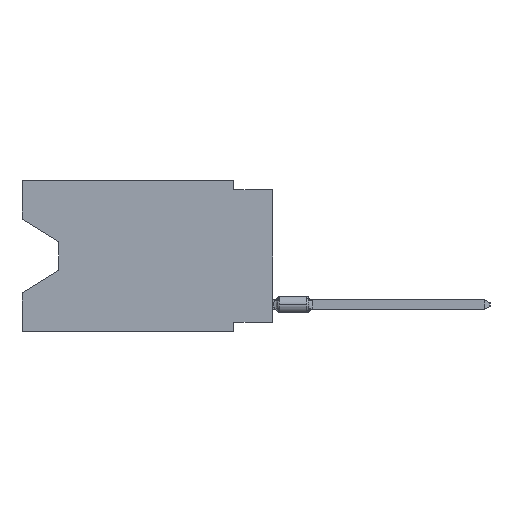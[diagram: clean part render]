
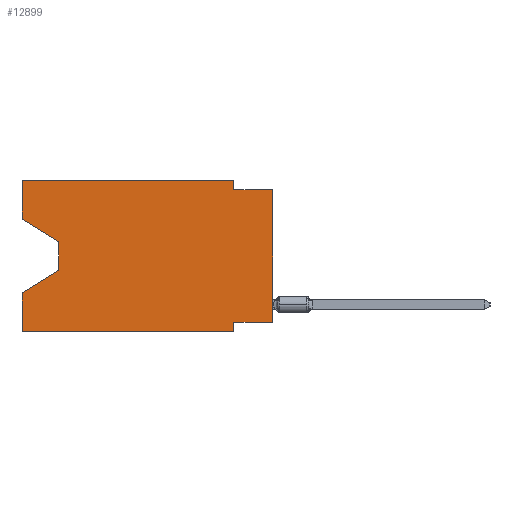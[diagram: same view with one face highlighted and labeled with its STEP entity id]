
A CAD part, left-side view. The second image highlights one B-rep face of the part: STEP entity #12899.
In plain terms, the highlighted planar face has unit normal (-1, 0, 0).
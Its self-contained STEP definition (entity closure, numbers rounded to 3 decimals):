
#1047 = LINE ( 'NONE', #26146, #38552 ) ;
#1642 = PLANE ( 'NONE',  #50426 ) ;
#1974 = VERTEX_POINT ( 'NONE', #61499 ) ;
#2406 = CARTESIAN_POINT ( 'NONE',  ( 0., 2.54, -0.635 ) ) ;
#3405 = VECTOR ( 'NONE', #42499, 1000. ) ;
#3642 = EDGE_CURVE ( 'NONE', #33038, #1974, #9113, .T. ) ;
#4799 = VECTOR ( 'NONE', #60959, 1000. ) ;
#5208 = EDGE_CURVE ( 'NONE', #33038, #33749, #40273, .T. ) ;
#6103 = DIRECTION ( 'NONE',  ( 0., 0., 1. ) ) ;
#6363 = EDGE_CURVE ( 'NONE', #18830, #42133, #46869, .T. ) ;
#9113 = LINE ( 'NONE', #77763, #74344 ) ;
#10353 = CARTESIAN_POINT ( 'NONE',  ( 0., 13.97, -4.013 ) ) ;
#10570 = CARTESIAN_POINT ( 'NONE',  ( 0., 2.54, 0. ) ) ;
#12063 = EDGE_CURVE ( 'NONE', #57108, #62061, #36703, .T. ) ;
#12899 = ADVANCED_FACE ( 'NONE', ( #32893 ), #1642, .F. ) ;
#14791 = CARTESIAN_POINT ( 'NONE',  ( 0., 0., 0. ) ) ;
#15684 = LINE ( 'NONE', #46924, #48604 ) ;
#17912 = DIRECTION ( 'NONE',  ( 0., 0., -1. ) ) ;
#18375 = CARTESIAN_POINT ( 'NONE',  ( 0., 0., -0.635 ) ) ;
#18619 = ORIENTED_EDGE ( 'NONE', *, *, #70072, .F. ) ;
#18830 = VERTEX_POINT ( 'NONE', #29238 ) ;
#19600 = ORIENTED_EDGE ( 'NONE', *, *, #3642, .F. ) ;
#20637 = ORIENTED_EDGE ( 'NONE', *, *, #6363, .F. ) ;
#20926 = CARTESIAN_POINT ( 'NONE',  ( 0., 16.383, -9.906 ) ) ;
#22497 = CARTESIAN_POINT ( 'NONE',  ( 0., 13.97, -5.893 ) ) ;
#22985 = DIRECTION ( 'NONE',  ( 0., 0., 1. ) ) ;
#23133 = EDGE_CURVE ( 'NONE', #42133, #64070, #15684, .T. ) ;
#26146 = CARTESIAN_POINT ( 'NONE',  ( 0., 13.97, -4.013 ) ) ;
#27724 = LINE ( 'NONE', #51567, #53513 ) ;
#28369 = DIRECTION ( 'NONE',  ( 0., -1., 0. ) ) ;
#29172 = EDGE_CURVE ( 'NONE', #62061, #59233, #1047, .T. ) ;
#29238 = CARTESIAN_POINT ( 'NONE',  ( 0., 16.383, 0. ) ) ;
#29783 = ORIENTED_EDGE ( 'NONE', *, *, #5208, .T. ) ;
#29927 = VECTOR ( 'NONE', #59141, 1000. ) ;
#29973 = LINE ( 'NONE', #79690, #62782 ) ;
#32835 = ORIENTED_EDGE ( 'NONE', *, *, #23133, .F. ) ;
#32893 = FACE_OUTER_BOUND ( 'NONE', #74694, .T. ) ;
#33038 = VERTEX_POINT ( 'NONE', #68652 ) ;
#33531 = ORIENTED_EDGE ( 'NONE', *, *, #44154, .T. ) ;
#33749 = VERTEX_POINT ( 'NONE', #44512 ) ;
#34199 = DIRECTION ( 'NONE',  ( 0., 1., 0. ) ) ;
#35881 = CARTESIAN_POINT ( 'NONE',  ( 0., 13.97, -5.893 ) ) ;
#36703 = LINE ( 'NONE', #67949, #73949 ) ;
#36957 = ORIENTED_EDGE ( 'NONE', *, *, #61454, .F. ) ;
#38552 = VECTOR ( 'NONE', #17912, 1000. ) ;
#40273 = LINE ( 'NONE', #14791, #41742 ) ;
#41742 = VECTOR ( 'NONE', #22985, 1000. ) ;
#42133 = VERTEX_POINT ( 'NONE', #10570 ) ;
#42499 = DIRECTION ( 'NONE',  ( 0., 0., 1. ) ) ;
#44154 = EDGE_CURVE ( 'NONE', #59233, #73232, #67120, .T. ) ;
#44512 = CARTESIAN_POINT ( 'NONE',  ( 0., 0., -0.635 ) ) ;
#45296 = ORIENTED_EDGE ( 'NONE', *, *, #77652, .F. ) ;
#46570 = VECTOR ( 'NONE', #68528, 1000. ) ;
#46869 = LINE ( 'NONE', #60811, #74651 ) ;
#46924 = CARTESIAN_POINT ( 'NONE',  ( 0., 2.54, 0. ) ) ;
#47840 = DIRECTION ( 'NONE',  ( 0., -0.855, -0.519 ) ) ;
#48604 = VECTOR ( 'NONE', #58873, 1000. ) ;
#49069 = CARTESIAN_POINT ( 'NONE',  ( 0., 16.383, 0. ) ) ;
#49210 = CARTESIAN_POINT ( 'NONE',  ( 0., 16.383, -2.546 ) ) ;
#50283 = CARTESIAN_POINT ( 'NONE',  ( 0., 2.54, -9.906 ) ) ;
#50426 = AXIS2_PLACEMENT_3D ( 'NONE', #72715, #59591, #60391 ) ;
#51496 = CARTESIAN_POINT ( 'NONE',  ( 0., 16.383, -7.36 ) ) ;
#51567 = CARTESIAN_POINT ( 'NONE',  ( 0., 2.54, -9.906 ) ) ;
#51763 = LINE ( 'NONE', #20926, #29927 ) ;
#52479 = ORIENTED_EDGE ( 'NONE', *, *, #68029, .F. ) ;
#52643 = ORIENTED_EDGE ( 'NONE', *, *, #79429, .T. ) ;
#53485 = VERTEX_POINT ( 'NONE', #50283 ) ;
#53513 = VECTOR ( 'NONE', #76641, 1000. ) ;
#53980 = ORIENTED_EDGE ( 'NONE', *, *, #12063, .T. ) ;
#55230 = LINE ( 'NONE', #49069, #3405 ) ;
#57108 = VERTEX_POINT ( 'NONE', #49210 ) ;
#58873 = DIRECTION ( 'NONE',  ( 0., 0., -1. ) ) ;
#59141 = DIRECTION ( 'NONE',  ( 0., -1., 0. ) ) ;
#59233 = VERTEX_POINT ( 'NONE', #22497 ) ;
#59591 = DIRECTION ( 'NONE',  ( 1., 0., 0. ) ) ;
#60391 = DIRECTION ( 'NONE',  ( 0., 0., -1. ) ) ;
#60811 = CARTESIAN_POINT ( 'NONE',  ( 0., 16.383, 0. ) ) ;
#60959 = DIRECTION ( 'NONE',  ( 0., 0.855, -0.519 ) ) ;
#61454 = EDGE_CURVE ( 'NONE', #63803, #73232, #29973, .T. ) ;
#61499 = CARTESIAN_POINT ( 'NONE',  ( 0., 2.54, -9.271 ) ) ;
#62061 = VERTEX_POINT ( 'NONE', #10353 ) ;
#62782 = VECTOR ( 'NONE', #6103, 1000. ) ;
#63803 = VERTEX_POINT ( 'NONE', #74051 ) ;
#64070 = VERTEX_POINT ( 'NONE', #2406 ) ;
#64844 = ORIENTED_EDGE ( 'NONE', *, *, #29172, .T. ) ;
#67120 = LINE ( 'NONE', #35881, #4799 ) ;
#67949 = CARTESIAN_POINT ( 'NONE',  ( 0., 16.383, -2.546 ) ) ;
#68029 = EDGE_CURVE ( 'NONE', #57108, #18830, #55230, .T. ) ;
#68528 = DIRECTION ( 'NONE',  ( 0., -1., 0. ) ) ;
#68652 = CARTESIAN_POINT ( 'NONE',  ( 0., 0., -9.271 ) ) ;
#70072 = EDGE_CURVE ( 'NONE', #1974, #53485, #27724, .T. ) ;
#72715 = CARTESIAN_POINT ( 'NONE',  ( 0., 16.383, 0. ) ) ;
#73232 = VERTEX_POINT ( 'NONE', #51496 ) ;
#73949 = VECTOR ( 'NONE', #47840, 1000. ) ;
#74051 = CARTESIAN_POINT ( 'NONE',  ( 0., 16.383, -9.906 ) ) ;
#74344 = VECTOR ( 'NONE', #34199, 1000. ) ;
#74651 = VECTOR ( 'NONE', #28369, 1000. ) ;
#74690 = LINE ( 'NONE', #18375, #46570 ) ;
#74694 = EDGE_LOOP ( 'NONE', ( #53980, #64844, #33531, #36957, #52643, #18619, #19600, #29783, #45296, #32835, #20637, #52479 ) ) ;
#76641 = DIRECTION ( 'NONE',  ( 0., 0., -1. ) ) ;
#77652 = EDGE_CURVE ( 'NONE', #64070, #33749, #74690, .T. ) ;
#77763 = CARTESIAN_POINT ( 'NONE',  ( 0., 0., -9.271 ) ) ;
#79429 = EDGE_CURVE ( 'NONE', #63803, #53485, #51763, .T. ) ;
#79690 = CARTESIAN_POINT ( 'NONE',  ( 0., 16.383, 0. ) ) ;
